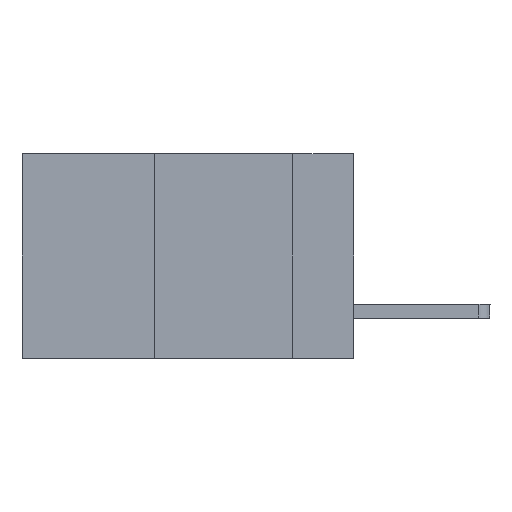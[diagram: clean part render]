
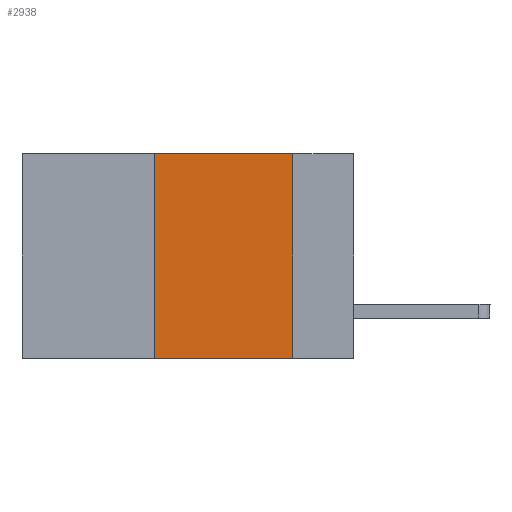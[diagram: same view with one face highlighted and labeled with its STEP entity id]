
A CAD part, left-side view. The second image highlights one B-rep face of the part: STEP entity #2938.
In plain terms, the highlighted planar face has unit normal (-1, 0, 0).
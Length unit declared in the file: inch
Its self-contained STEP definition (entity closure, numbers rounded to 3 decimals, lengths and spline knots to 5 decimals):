
#118 = EDGE_LOOP ( 'NONE', ( #9448, #1008, #843, #8486 ) ) ;
#247 = DIRECTION ( 'NONE',  ( 0., 0., 1. ) ) ;
#382 = DIRECTION ( 'NONE',  ( 0., 0., -1. ) ) ;
#503 = DIRECTION ( 'NONE',  ( 0., 0., -1. ) ) ;
#843 = ORIENTED_EDGE ( 'NONE', *, *, #3597, .F. ) ;
#1008 = ORIENTED_EDGE ( 'NONE', *, *, #6881, .F. ) ;
#1053 = PLANE ( 'NONE',  #6265 ) ;
#1111 = VECTOR ( 'NONE', #503, 39.37008 ) ;
#1290 = VECTOR ( 'NONE', #247, 39.37008 ) ;
#1780 = VERTEX_POINT ( 'NONE', #2872 ) ;
#1860 = CARTESIAN_POINT ( 'NONE',  ( 0., 0.36, 0. ) ) ;
#2201 = FACE_OUTER_BOUND ( 'NONE', #118, .T. ) ;
#2293 = DIRECTION ( 'NONE',  ( 0., -1., 0. ) ) ;
#2576 = CARTESIAN_POINT ( 'NONE',  ( 0., 0.11, -0.37 ) ) ;
#2693 = CARTESIAN_POINT ( 'NONE',  ( 0., 0.6, 0. ) ) ;
#2735 = VERTEX_POINT ( 'NONE', #3316 ) ;
#2872 = CARTESIAN_POINT ( 'NONE',  ( 0., 0.11, 0. ) ) ;
#2938 = ADVANCED_FACE ( 'NONE', ( #2201 ), #1053, .F. ) ;
#3112 = VECTOR ( 'NONE', #2293, 39.37008 ) ;
#3285 = LINE ( 'NONE', #7984, #1111 ) ;
#3316 = CARTESIAN_POINT ( 'NONE',  ( 0., 0.36, -0.37 ) ) ;
#3597 = EDGE_CURVE ( 'NONE', #2735, #8874, #5655, .T. ) ;
#3756 = LINE ( 'NONE', #3949, #3112 ) ;
#3949 = CARTESIAN_POINT ( 'NONE',  ( 0., 0.6, 0. ) ) ;
#4074 = CARTESIAN_POINT ( 'NONE',  ( 0., 0.6, -0.37 ) ) ;
#4468 = DIRECTION ( 'NONE',  ( 1., 0., 0. ) ) ;
#5085 = EDGE_CURVE ( 'NONE', #1780, #9233, #3285, .T. ) ;
#5655 = LINE ( 'NONE', #1860, #1290 ) ;
#6130 = LINE ( 'NONE', #4074, #7697 ) ;
#6265 = AXIS2_PLACEMENT_3D ( 'NONE', #2693, #4468, #382 ) ;
#6881 = EDGE_CURVE ( 'NONE', #8874, #1780, #3756, .T. ) ;
#7061 = CARTESIAN_POINT ( 'NONE',  ( 0., 0.36, 0. ) ) ;
#7697 = VECTOR ( 'NONE', #8230, 39.37008 ) ;
#7984 = CARTESIAN_POINT ( 'NONE',  ( 0., 0.11, 0. ) ) ;
#8230 = DIRECTION ( 'NONE',  ( 0., -1., 0. ) ) ;
#8486 = ORIENTED_EDGE ( 'NONE', *, *, #9170, .T. ) ;
#8874 = VERTEX_POINT ( 'NONE', #7061 ) ;
#9170 = EDGE_CURVE ( 'NONE', #2735, #9233, #6130, .T. ) ;
#9233 = VERTEX_POINT ( 'NONE', #2576 ) ;
#9448 = ORIENTED_EDGE ( 'NONE', *, *, #5085, .F. ) ;
